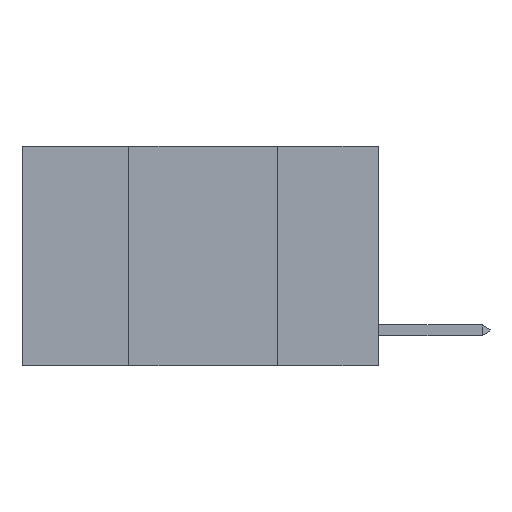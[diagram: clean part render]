
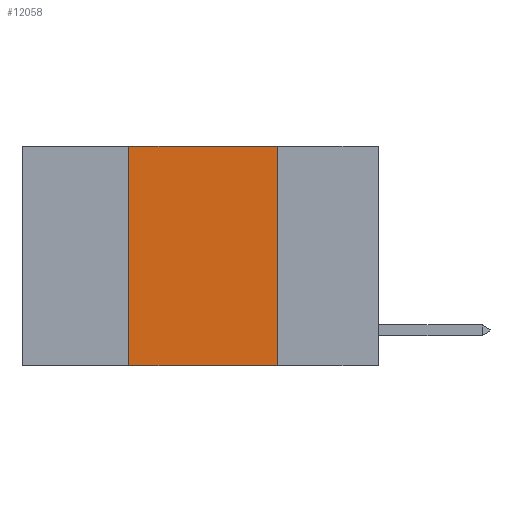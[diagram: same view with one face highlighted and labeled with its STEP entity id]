
A CAD part, left-side view. The second image highlights one B-rep face of the part: STEP entity #12058.
In plain terms, the highlighted planar face has unit normal (-1, 0, 0).
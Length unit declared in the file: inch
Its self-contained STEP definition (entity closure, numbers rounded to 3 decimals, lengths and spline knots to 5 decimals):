
#363 = LINE ( 'NONE', #7046, #9530 ) ;
#1762 = ORIENTED_EDGE ( 'NONE', *, *, #16305, .T. ) ;
#2359 = VECTOR ( 'NONE', #6536, 39.37008 ) ;
#2692 = ORIENTED_EDGE ( 'NONE', *, *, #24081, .F. ) ;
#2884 = CARTESIAN_POINT ( 'NONE',  ( 0., 0.42, -0.37 ) ) ;
#3589 = ORIENTED_EDGE ( 'NONE', *, *, #21430, .F. ) ;
#4177 = VERTEX_POINT ( 'NONE', #9508 ) ;
#5819 = CARTESIAN_POINT ( 'NONE',  ( 0., 0.17, 0. ) ) ;
#5973 = PLANE ( 'NONE',  #21252 ) ;
#6536 = DIRECTION ( 'NONE',  ( 0., -1., 0. ) ) ;
#7046 = CARTESIAN_POINT ( 'NONE',  ( 0., 0.42, 0. ) ) ;
#8071 = CARTESIAN_POINT ( 'NONE',  ( 0., 0.6, 0. ) ) ;
#8797 = CARTESIAN_POINT ( 'NONE',  ( 0., 0.6, 0. ) ) ;
#9147 = VERTEX_POINT ( 'NONE', #5819 ) ;
#9285 = ORIENTED_EDGE ( 'NONE', *, *, #11613, .F. ) ;
#9508 = CARTESIAN_POINT ( 'NONE',  ( 0., 0.42, 0. ) ) ;
#9530 = VECTOR ( 'NONE', #15068, 39.37008 ) ;
#11613 = EDGE_CURVE ( 'NONE', #9147, #16848, #11958, .T. ) ;
#11958 = LINE ( 'NONE', #16441, #23030 ) ;
#12058 = ADVANCED_FACE ( 'NONE', ( #18746 ), #5973, .F. ) ;
#12501 = DIRECTION ( 'NONE',  ( 0., 0., -1. ) ) ;
#12792 = DIRECTION ( 'NONE',  ( 0., -1., 0. ) ) ;
#13987 = VERTEX_POINT ( 'NONE', #2884 ) ;
#14759 = LINE ( 'NONE', #18969, #20473 ) ;
#15068 = DIRECTION ( 'NONE',  ( 0., 0., 1. ) ) ;
#15393 = LINE ( 'NONE', #8797, #2359 ) ;
#16305 = EDGE_CURVE ( 'NONE', #13987, #16848, #14759, .T. ) ;
#16441 = CARTESIAN_POINT ( 'NONE',  ( 0., 0.17, 0. ) ) ;
#16848 = VERTEX_POINT ( 'NONE', #24002 ) ;
#17618 = DIRECTION ( 'NONE',  ( 0., 0., -1. ) ) ;
#18746 = FACE_OUTER_BOUND ( 'NONE', #25880, .T. ) ;
#18969 = CARTESIAN_POINT ( 'NONE',  ( 0., 0.6, -0.37 ) ) ;
#20473 = VECTOR ( 'NONE', #12792, 39.37008 ) ;
#21252 = AXIS2_PLACEMENT_3D ( 'NONE', #8071, #25231, #17618 ) ;
#21430 = EDGE_CURVE ( 'NONE', #4177, #9147, #15393, .T. ) ;
#23030 = VECTOR ( 'NONE', #12501, 39.37008 ) ;
#24002 = CARTESIAN_POINT ( 'NONE',  ( 0., 0.17, -0.37 ) ) ;
#24081 = EDGE_CURVE ( 'NONE', #13987, #4177, #363, .T. ) ;
#25231 = DIRECTION ( 'NONE',  ( 1., 0., 0. ) ) ;
#25880 = EDGE_LOOP ( 'NONE', ( #9285, #3589, #2692, #1762 ) ) ;
